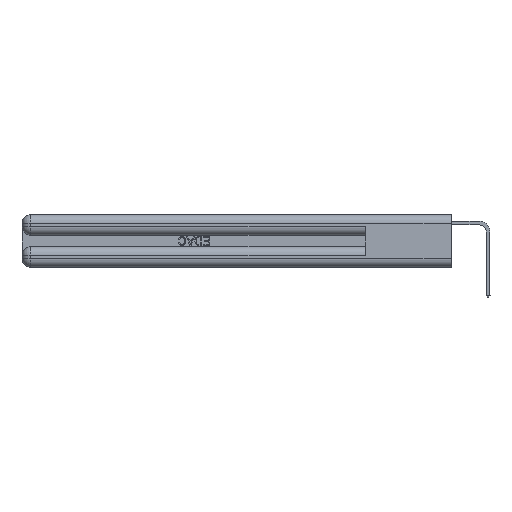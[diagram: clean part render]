
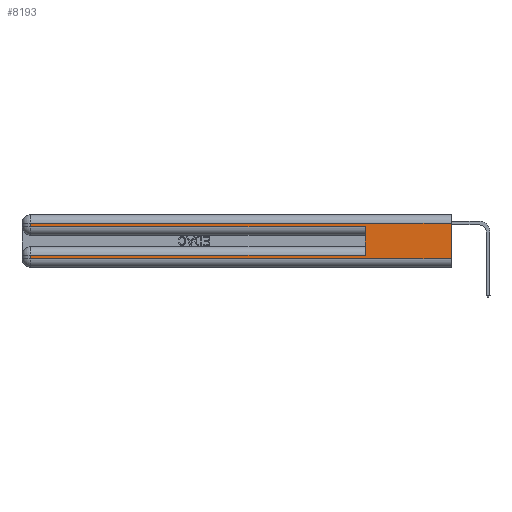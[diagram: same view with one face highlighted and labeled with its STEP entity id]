
A CAD part, left-side view. The second image highlights one B-rep face of the part: STEP entity #8193.
In plain terms, the highlighted planar face has unit normal (-1, 0, 0).
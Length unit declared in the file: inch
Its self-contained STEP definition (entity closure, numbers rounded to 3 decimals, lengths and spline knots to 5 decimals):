
#86 = CARTESIAN_POINT ( 'NONE',  ( 0., 0.6, 0.285 ) ) ;
#229 = DIRECTION ( 'NONE',  ( 0., 0., -1. ) ) ;
#510 = VERTEX_POINT ( 'NONE', #86 ) ;
#514 = CARTESIAN_POINT ( 'NONE',  ( 0., 0., 0.37 ) ) ;
#797 = LINE ( 'NONE', #22248, #14917 ) ;
#2546 = VERTEX_POINT ( 'NONE', #20830 ) ;
#2739 = DIRECTION ( 'NONE',  ( 0., 0., -1. ) ) ;
#2920 = VERTEX_POINT ( 'NONE', #19352 ) ;
#2970 = VERTEX_POINT ( 'NONE', #10810 ) ;
#3116 = ORIENTED_EDGE ( 'NONE', *, *, #18557, .T. ) ;
#3246 = DIRECTION ( 'NONE',  ( 0., 1., 0. ) ) ;
#4220 = PLANE ( 'NONE',  #30446 ) ;
#4940 = LINE ( 'NONE', #514, #16327 ) ;
#5089 = LINE ( 'NONE', #14747, #10190 ) ;
#5425 = CARTESIAN_POINT ( 'NONE',  ( 0., 0., 0.085 ) ) ;
#5821 = ORIENTED_EDGE ( 'NONE', *, *, #12263, .F. ) ;
#6093 = ORIENTED_EDGE ( 'NONE', *, *, #24623, .T. ) ;
#6258 = LINE ( 'NONE', #9226, #15406 ) ;
#6712 = EDGE_CURVE ( 'NONE', #2546, #20975, #7727, .T. ) ;
#7727 = LINE ( 'NONE', #5425, #26996 ) ;
#8193 = ADVANCED_FACE ( 'NONE', ( #11246 ), #4220, .F. ) ;
#8231 = VERTEX_POINT ( 'NONE', #30515 ) ;
#9226 = CARTESIAN_POINT ( 'NONE',  ( 0., 2.94, 0.37 ) ) ;
#9458 = VERTEX_POINT ( 'NONE', #12668 ) ;
#9920 = ORIENTED_EDGE ( 'NONE', *, *, #6712, .T. ) ;
#10190 = VECTOR ( 'NONE', #24043, 39.37008 ) ;
#10810 = CARTESIAN_POINT ( 'NONE',  ( 0., 2.94, 0.31 ) ) ;
#11246 = FACE_OUTER_BOUND ( 'NONE', #24733, .T. ) ;
#12263 = EDGE_CURVE ( 'NONE', #2546, #510, #797, .T. ) ;
#12668 = CARTESIAN_POINT ( 'NONE',  ( 0., 0., 0.31 ) ) ;
#12996 = EDGE_CURVE ( 'NONE', #9458, #8231, #4940, .T. ) ;
#13395 = ORIENTED_EDGE ( 'NONE', *, *, #27460, .T. ) ;
#14284 = CARTESIAN_POINT ( 'NONE',  ( 0., 2.94, 0.285 ) ) ;
#14649 = ORIENTED_EDGE ( 'NONE', *, *, #20479, .T. ) ;
#14747 = CARTESIAN_POINT ( 'NONE',  ( 0., 0., 0.31 ) ) ;
#14791 = ORIENTED_EDGE ( 'NONE', *, *, #26000, .T. ) ;
#14917 = VECTOR ( 'NONE', #26808, 39.37008 ) ;
#15406 = VECTOR ( 'NONE', #16253, 39.37008 ) ;
#15748 = VECTOR ( 'NONE', #17425, 39.37008 ) ;
#16218 = DIRECTION ( 'NONE',  ( 1., 0., 0. ) ) ;
#16253 = DIRECTION ( 'NONE',  ( 0., 0., -1. ) ) ;
#16327 = VECTOR ( 'NONE', #229, 39.37008 ) ;
#17289 = LINE ( 'NONE', #19573, #15748 ) ;
#17425 = DIRECTION ( 'NONE',  ( 0., -1., 0. ) ) ;
#18557 = EDGE_CURVE ( 'NONE', #21699, #510, #17289, .T. ) ;
#19032 = CARTESIAN_POINT ( 'NONE',  ( 0., 2.94, 0.085 ) ) ;
#19352 = CARTESIAN_POINT ( 'NONE',  ( 0., 2.94, 0.06 ) ) ;
#19573 = CARTESIAN_POINT ( 'NONE',  ( 0., 0., 0.285 ) ) ;
#20455 = DIRECTION ( 'NONE',  ( 0., -1., 0. ) ) ;
#20479 = EDGE_CURVE ( 'NONE', #20975, #2920, #26839, .T. ) ;
#20830 = CARTESIAN_POINT ( 'NONE',  ( 0., 0.6, 0.085 ) ) ;
#20975 = VERTEX_POINT ( 'NONE', #19032 ) ;
#21699 = VERTEX_POINT ( 'NONE', #14284 ) ;
#22248 = CARTESIAN_POINT ( 'NONE',  ( 0., 0.6, 0.145 ) ) ;
#24043 = DIRECTION ( 'NONE',  ( 0., 1., 0. ) ) ;
#24623 = EDGE_CURVE ( 'NONE', #2920, #8231, #25753, .T. ) ;
#24733 = EDGE_LOOP ( 'NONE', ( #27435, #14791, #13395, #3116, #5821, #9920, #14649, #6093 ) ) ;
#25354 = DIRECTION ( 'NONE',  ( 0., 0., -1. ) ) ;
#25753 = LINE ( 'NONE', #27987, #30066 ) ;
#26000 = EDGE_CURVE ( 'NONE', #9458, #2970, #5089, .T. ) ;
#26537 = CARTESIAN_POINT ( 'NONE',  ( 0., 2.94, 0.37 ) ) ;
#26808 = DIRECTION ( 'NONE',  ( 0., 0., 1. ) ) ;
#26839 = LINE ( 'NONE', #26537, #30401 ) ;
#26996 = VECTOR ( 'NONE', #3246, 39.37008 ) ;
#27435 = ORIENTED_EDGE ( 'NONE', *, *, #12996, .F. ) ;
#27460 = EDGE_CURVE ( 'NONE', #2970, #21699, #6258, .T. ) ;
#27713 = CARTESIAN_POINT ( 'NONE',  ( 0., 0., 0.37 ) ) ;
#27987 = CARTESIAN_POINT ( 'NONE',  ( 0., 0., 0.06 ) ) ;
#30066 = VECTOR ( 'NONE', #20455, 39.37008 ) ;
#30401 = VECTOR ( 'NONE', #2739, 39.37008 ) ;
#30446 = AXIS2_PLACEMENT_3D ( 'NONE', #27713, #16218, #25354 ) ;
#30515 = CARTESIAN_POINT ( 'NONE',  ( 0., 0., 0.06 ) ) ;
